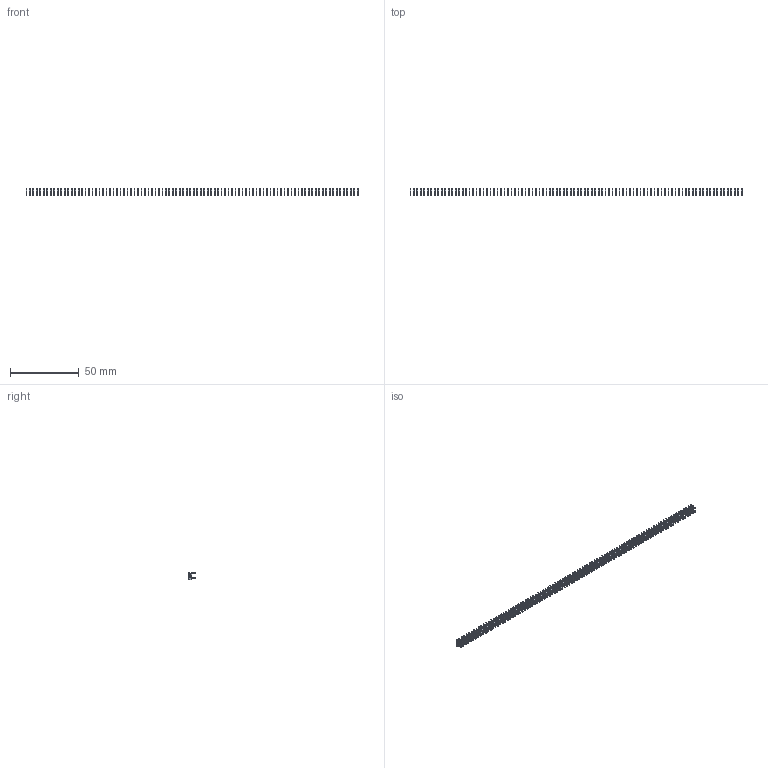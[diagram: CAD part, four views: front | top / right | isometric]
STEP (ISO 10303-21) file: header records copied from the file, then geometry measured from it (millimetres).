
FILE_DESCRIPTION (( 'STEP AP203' ), '1' );
FILE_NAME ('105-096-208-100.STEP', '2020-04-08T01:15:40', ( '' ), ( '' ), 'SwSTEP 2.0', 'SolidWorks 2016', '' );
FILE_SCHEMA (( 'CONFIG_CONTROL_DESIGN' ));
Length unit declared in the file: inch
Products named in the file (2): 100-290-001_100-290-208; 105-096-208-100
Assembly tree (96 placements, depth 2):
  105-096-208-100
    100-290-001_100-290-208  x96
Bounding box: 241.81 x 4.83 x 5.17 mm (x, y, z)
Volume: 660.5 mm3; surface area: 4079.6 mm2
Topology: 96 solids, 96 shells, 2400 faces, 6624 edges, 4416 vertices
Faces by surface type: plane 2112, cylinder 288
Entity records: 4029 total; most frequent: DIRECTION 323, CARTESIAN_POINT 239, DATE_AND_TIME 202, COORDINATED_UNIVERSAL_TIME_OFFSET 202, LOCAL_TIME 202, CALENDAR_DATE 202, ORIENTED_EDGE 138, AXIS2_PLACEMENT_3D 130
